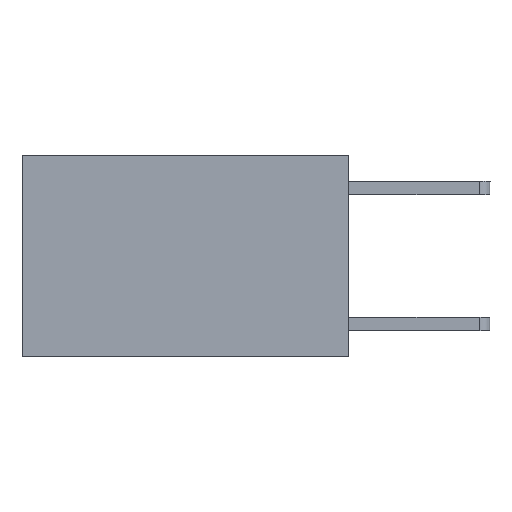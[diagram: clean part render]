
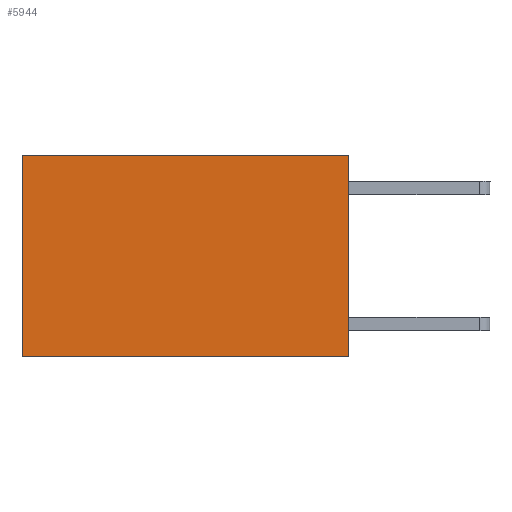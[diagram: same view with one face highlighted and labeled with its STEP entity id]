
A CAD part, left-side view. The second image highlights one B-rep face of the part: STEP entity #5944.
In plain terms, the highlighted planar face has unit normal (-1, 0, 0).
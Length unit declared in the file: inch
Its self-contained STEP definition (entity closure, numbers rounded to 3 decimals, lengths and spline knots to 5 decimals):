
#98 = CARTESIAN_POINT ( 'NONE',  ( 0.2625, 0., -0.37 ) ) ;
#99 = ORIENTED_EDGE ( 'NONE', *, *, #732, .T. ) ;
#568 = CARTESIAN_POINT ( 'NONE',  ( 0.2625, 0.6, 0. ) ) ;
#620 = DIRECTION ( 'NONE',  ( 0., 0., -1. ) ) ;
#637 = ORIENTED_EDGE ( 'NONE', *, *, #7569, .F. ) ;
#694 = VECTOR ( 'NONE', #3188, 39.37008 ) ;
#732 = EDGE_CURVE ( 'NONE', #3739, #2006, #2533, .T. ) ;
#801 = ORIENTED_EDGE ( 'NONE', *, *, #6360, .T. ) ;
#806 = VERTEX_POINT ( 'NONE', #98 ) ;
#858 = VECTOR ( 'NONE', #7419, 39.37008 ) ;
#909 = LINE ( 'NONE', #6496, #694 ) ;
#1033 = VECTOR ( 'NONE', #7859, 39.37008 ) ;
#1287 = LINE ( 'NONE', #6808, #1033 ) ;
#1850 = CARTESIAN_POINT ( 'NONE',  ( 0.2625, 0., 0. ) ) ;
#2006 = VERTEX_POINT ( 'NONE', #2873 ) ;
#2533 = LINE ( 'NONE', #4941, #858 ) ;
#2699 = CARTESIAN_POINT ( 'NONE',  ( 0.2625, 0.6, -0.37 ) ) ;
#2873 = CARTESIAN_POINT ( 'NONE',  ( 0.2625, 0.6, 0. ) ) ;
#3188 = DIRECTION ( 'NONE',  ( 0., 0., -1. ) ) ;
#3739 = VERTEX_POINT ( 'NONE', #5076 ) ;
#4146 = VERTEX_POINT ( 'NONE', #2699 ) ;
#4209 = EDGE_CURVE ( 'NONE', #806, #4146, #1287, .T. ) ;
#4390 = DIRECTION ( 'NONE',  ( 0., 0., -1. ) ) ;
#4774 = PLANE ( 'NONE',  #6627 ) ;
#4941 = CARTESIAN_POINT ( 'NONE',  ( 0.2625, 0., 0. ) ) ;
#5076 = CARTESIAN_POINT ( 'NONE',  ( 0.2625, 0., 0. ) ) ;
#5600 = VECTOR ( 'NONE', #620, 39.37008 ) ;
#5608 = LINE ( 'NONE', #568, #5600 ) ;
#5683 = DIRECTION ( 'NONE',  ( 1., 0., 0. ) ) ;
#5932 = EDGE_LOOP ( 'NONE', ( #801, #5975, #637, #99 ) ) ;
#5944 = ADVANCED_FACE ( 'NONE', ( #6689 ), #4774, .F. ) ;
#5975 = ORIENTED_EDGE ( 'NONE', *, *, #4209, .F. ) ;
#6360 = EDGE_CURVE ( 'NONE', #2006, #4146, #5608, .T. ) ;
#6496 = CARTESIAN_POINT ( 'NONE',  ( 0.2625, 0., 0. ) ) ;
#6627 = AXIS2_PLACEMENT_3D ( 'NONE', #1850, #5683, #4390 ) ;
#6689 = FACE_OUTER_BOUND ( 'NONE', #5932, .T. ) ;
#6808 = CARTESIAN_POINT ( 'NONE',  ( 0.2625, 0., -0.37 ) ) ;
#7419 = DIRECTION ( 'NONE',  ( 0., 1., 0. ) ) ;
#7569 = EDGE_CURVE ( 'NONE', #3739, #806, #909, .T. ) ;
#7859 = DIRECTION ( 'NONE',  ( 0., 1., 0. ) ) ;
